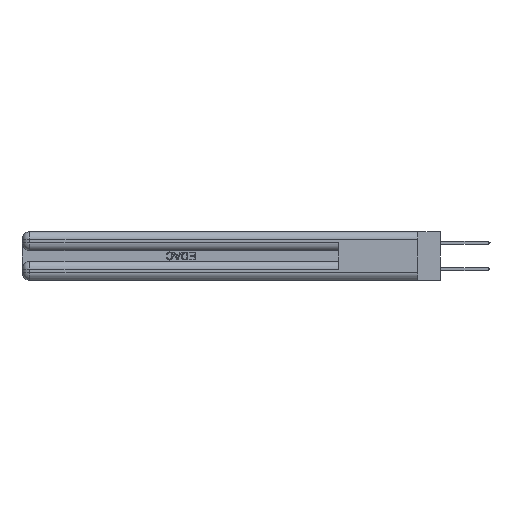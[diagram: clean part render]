
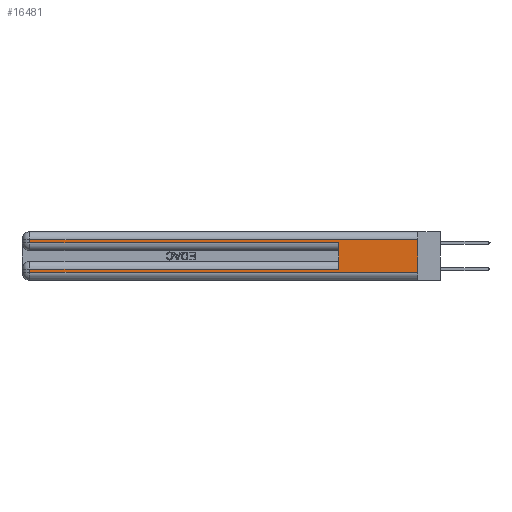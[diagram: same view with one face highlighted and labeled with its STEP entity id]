
A CAD part, left-side view. The second image highlights one B-rep face of the part: STEP entity #16481.
In plain terms, the highlighted planar face has unit normal (-1, 0, 0).
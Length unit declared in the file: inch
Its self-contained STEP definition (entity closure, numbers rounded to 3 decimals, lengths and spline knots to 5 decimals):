
#1395 = DIRECTION ( 'NONE',  ( 0., 0., -1. ) ) ;
#1876 = LINE ( 'NONE', #27566, #31498 ) ;
#2594 = DIRECTION ( 'NONE',  ( 1., 0., 0. ) ) ;
#4647 = ORIENTED_EDGE ( 'NONE', *, *, #19564, .T. ) ;
#4809 = ORIENTED_EDGE ( 'NONE', *, *, #39506, .F. ) ;
#4910 = LINE ( 'NONE', #37818, #32076 ) ;
#6740 = CARTESIAN_POINT ( 'NONE',  ( 0., 0., 0.285 ) ) ;
#6741 = LINE ( 'NONE', #31385, #9761 ) ;
#6893 = EDGE_CURVE ( 'NONE', #21023, #39702, #19060, .T. ) ;
#7505 = VERTEX_POINT ( 'NONE', #21349 ) ;
#8295 = DIRECTION ( 'NONE',  ( 0., 0., -1. ) ) ;
#9761 = VECTOR ( 'NONE', #8295, 39.37008 ) ;
#10069 = ORIENTED_EDGE ( 'NONE', *, *, #21417, .T. ) ;
#11499 = ORIENTED_EDGE ( 'NONE', *, *, #34882, .T. ) ;
#11736 = VERTEX_POINT ( 'NONE', #47352 ) ;
#13809 = ORIENTED_EDGE ( 'NONE', *, *, #6893, .F. ) ;
#13955 = EDGE_CURVE ( 'NONE', #46830, #33782, #49168, .T. ) ;
#13992 = AXIS2_PLACEMENT_3D ( 'NONE', #25941, #2594, #21883 ) ;
#14698 = DIRECTION ( 'NONE',  ( 0., 1., 0. ) ) ;
#14736 = DIRECTION ( 'NONE',  ( 0., 1., 0. ) ) ;
#15519 = ORIENTED_EDGE ( 'NONE', *, *, #13955, .T. ) ;
#16257 = DIRECTION ( 'NONE',  ( 0., 0., -1. ) ) ;
#16481 = ADVANCED_FACE ( 'NONE', ( #17261 ), #44923, .F. ) ;
#17261 = FACE_OUTER_BOUND ( 'NONE', #37383, .T. ) ;
#18348 = CARTESIAN_POINT ( 'NONE',  ( 0., 0., 0.06 ) ) ;
#19060 = LINE ( 'NONE', #21063, #45588 ) ;
#19183 = VECTOR ( 'NONE', #21806, 39.37008 ) ;
#19564 = EDGE_CURVE ( 'NONE', #33782, #7505, #6741, .T. ) ;
#21023 = VERTEX_POINT ( 'NONE', #23698 ) ;
#21026 = EDGE_CURVE ( 'NONE', #39311, #27029, #1876, .T. ) ;
#21063 = CARTESIAN_POINT ( 'NONE',  ( 0., 0., 0.37 ) ) ;
#21080 = CARTESIAN_POINT ( 'NONE',  ( 0., 0.6, 0.145 ) ) ;
#21349 = CARTESIAN_POINT ( 'NONE',  ( 0., 2.94, 0.06 ) ) ;
#21417 = EDGE_CURVE ( 'NONE', #21023, #39311, #4910, .T. ) ;
#21806 = DIRECTION ( 'NONE',  ( 0., -1., 0. ) ) ;
#21883 = DIRECTION ( 'NONE',  ( 0., 0., -1. ) ) ;
#23698 = CARTESIAN_POINT ( 'NONE',  ( 0., 0., 0.31 ) ) ;
#25941 = CARTESIAN_POINT ( 'NONE',  ( 0., 0., 0.37 ) ) ;
#27029 = VERTEX_POINT ( 'NONE', #37202 ) ;
#27381 = ORIENTED_EDGE ( 'NONE', *, *, #21026, .T. ) ;
#27566 = CARTESIAN_POINT ( 'NONE',  ( 0., 2.94, 0.37 ) ) ;
#27972 = CARTESIAN_POINT ( 'NONE',  ( 0., 2.94, 0.31 ) ) ;
#31385 = CARTESIAN_POINT ( 'NONE',  ( 0., 2.94, 0.37 ) ) ;
#31498 = VECTOR ( 'NONE', #16257, 39.37008 ) ;
#32076 = VECTOR ( 'NONE', #14698, 39.37008 ) ;
#32864 = VECTOR ( 'NONE', #14736, 39.37008 ) ;
#33063 = LINE ( 'NONE', #6740, #19183 ) ;
#33782 = VERTEX_POINT ( 'NONE', #43775 ) ;
#34882 = EDGE_CURVE ( 'NONE', #7505, #39702, #41742, .T. ) ;
#35908 = DIRECTION ( 'NONE',  ( 0., 0., 1. ) ) ;
#37202 = CARTESIAN_POINT ( 'NONE',  ( 0., 2.94, 0.285 ) ) ;
#37383 = EDGE_LOOP ( 'NONE', ( #13809, #10069, #27381, #46870, #4809, #15519, #4647, #11499 ) ) ;
#37679 = DIRECTION ( 'NONE',  ( 0., -1., 0. ) ) ;
#37818 = CARTESIAN_POINT ( 'NONE',  ( 0., 0., 0.31 ) ) ;
#38160 = CARTESIAN_POINT ( 'NONE',  ( 0., 0., 0.06 ) ) ;
#39311 = VERTEX_POINT ( 'NONE', #27972 ) ;
#39506 = EDGE_CURVE ( 'NONE', #46830, #11736, #46749, .T. ) ;
#39702 = VERTEX_POINT ( 'NONE', #18348 ) ;
#41348 = CARTESIAN_POINT ( 'NONE',  ( 0., 0., 0.085 ) ) ;
#41742 = LINE ( 'NONE', #38160, #42318 ) ;
#42136 = CARTESIAN_POINT ( 'NONE',  ( 0., 0.6, 0.085 ) ) ;
#42318 = VECTOR ( 'NONE', #37679, 39.37008 ) ;
#43775 = CARTESIAN_POINT ( 'NONE',  ( 0., 2.94, 0.085 ) ) ;
#44684 = EDGE_CURVE ( 'NONE', #27029, #11736, #33063, .T. ) ;
#44923 = PLANE ( 'NONE',  #13992 ) ;
#45588 = VECTOR ( 'NONE', #1395, 39.37008 ) ;
#46103 = VECTOR ( 'NONE', #35908, 39.37008 ) ;
#46749 = LINE ( 'NONE', #21080, #46103 ) ;
#46830 = VERTEX_POINT ( 'NONE', #42136 ) ;
#46870 = ORIENTED_EDGE ( 'NONE', *, *, #44684, .T. ) ;
#47352 = CARTESIAN_POINT ( 'NONE',  ( 0., 0.6, 0.285 ) ) ;
#49168 = LINE ( 'NONE', #41348, #32864 ) ;
